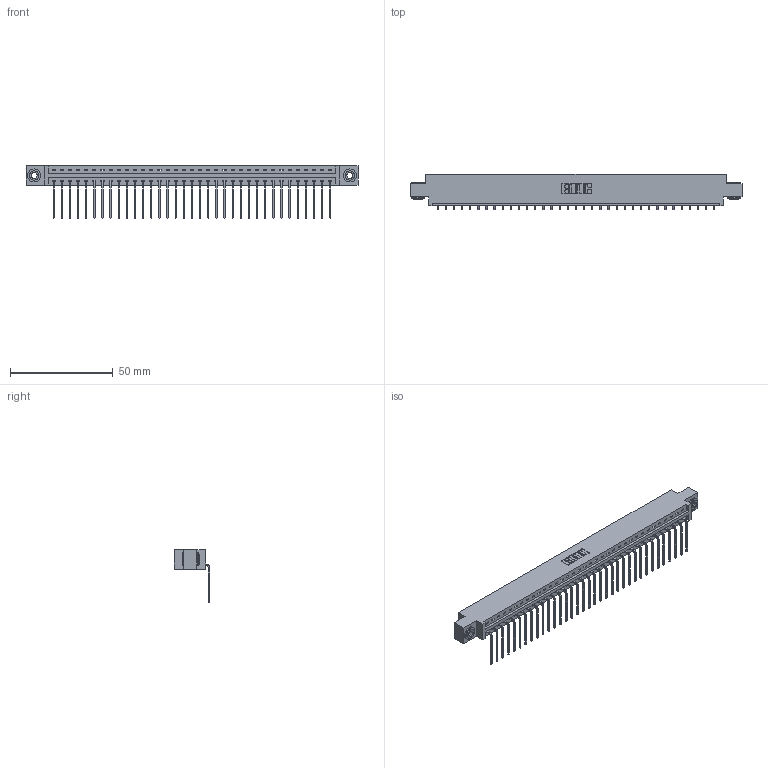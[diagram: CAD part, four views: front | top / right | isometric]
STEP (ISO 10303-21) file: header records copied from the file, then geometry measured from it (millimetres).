
FILE_DESCRIPTION (( 'STEP AP203' ), '1' );
FILE_NAME ('337-035-559-603.STEP', '2018-08-07T21:15:01', ( '' ), ( '' ), 'SwSTEP 2.0', 'SolidWorks 2016', '' );
FILE_SCHEMA (( 'CONFIG_CONTROL_DESIGN' ));
Length unit declared in the file: inch
Products named in the file (4): 345-292-001_558 559 Tail - 1; 345-250-002_345-250-002-102; 337-035-559-603; 337 Part_0.170 Offset - 0.156 Dia-TH
Assembly tree (38 placements, depth 2):
  337-035-559-603
    337 Part_0.170 Offset - 0.156 Dia-TH
    345-292-001_558 559 Tail - 1  x35
    345-250-002_345-250-002-102  x2
Bounding box: 161.7 x 17.09 x 25.53 mm (x, y, z)
Volume: 16736.5 mm3; surface area: 18301.4 mm2
Topology: 38 solids, 38 shells, 2396 faces, 7189 edges, 4742 vertices
Faces by surface type: plane 1764, cylinder 624, cone 8
Entity records: 27788 total; most frequent: CARTESIAN_POINT 4818, ORIENTED_EDGE 4782, DIRECTION 4103, EDGE_CURVE 2391, LINE 2239, VECTOR 2239, VERTEX_POINT 1590, AXIS2_PLACEMENT_3D 932
